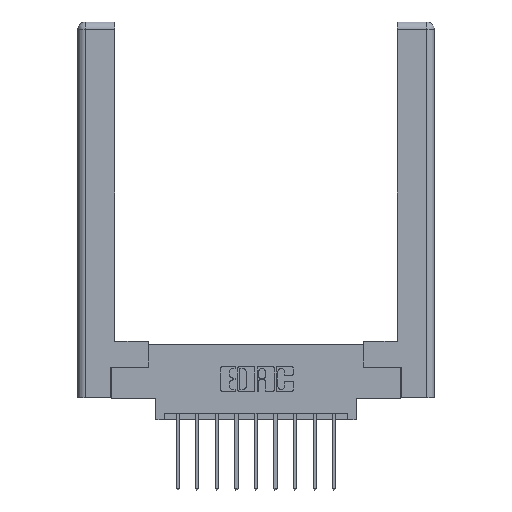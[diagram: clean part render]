
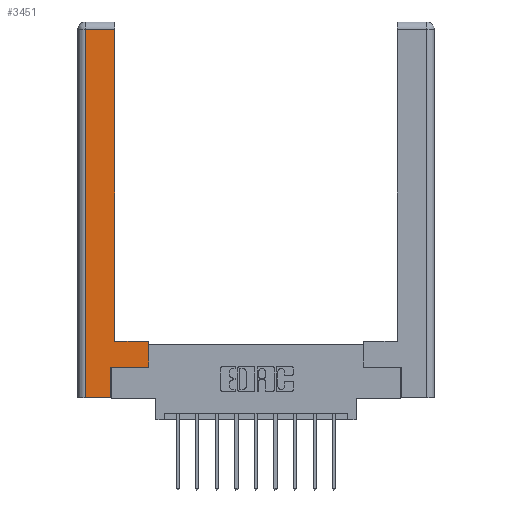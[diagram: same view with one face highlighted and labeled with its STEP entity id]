
A CAD part, top view. The second image highlights one B-rep face of the part: STEP entity #3451.
In plain terms, the highlighted planar face has unit normal (0, 0, 1).
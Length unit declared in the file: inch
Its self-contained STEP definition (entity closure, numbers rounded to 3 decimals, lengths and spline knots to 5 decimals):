
#70 = ORIENTED_EDGE ( 'NONE', *, *, #8937, .T. ) ;
#324 = FACE_OUTER_BOUND ( 'NONE', #2742, .T. ) ;
#689 = PLANE ( 'NONE',  #3331 ) ;
#798 = CARTESIAN_POINT ( 'NONE',  ( 0.295, 0.45, 0. ) ) ;
#870 = ORIENTED_EDGE ( 'NONE', *, *, #9145, .T. ) ;
#1037 = ORIENTED_EDGE ( 'NONE', *, *, #11974, .T. ) ;
#1301 = CARTESIAN_POINT ( 'NONE',  ( 0.565, 0.245, 0. ) ) ;
#1412 = VECTOR ( 'NONE', #5843, 39.37008 ) ;
#1646 = CARTESIAN_POINT ( 'NONE',  ( 0., 0., 0. ) ) ;
#2191 = DIRECTION ( 'NONE',  ( -1., 0., 0. ) ) ;
#2213 = DIRECTION ( 'NONE',  ( -1., 0., 0. ) ) ;
#2419 = LINE ( 'NONE', #10620, #13935 ) ;
#2433 = LINE ( 'NONE', #7003, #1412 ) ;
#2742 = EDGE_LOOP ( 'NONE', ( #870, #13878, #9900, #4125, #12414, #70, #5429, #1037 ) ) ;
#2788 = DIRECTION ( 'NONE',  ( 0., 0., -1. ) ) ;
#3029 = EDGE_CURVE ( 'NONE', #13375, #9802, #7976, .T. ) ;
#3331 = AXIS2_PLACEMENT_3D ( 'NONE', #1646, #2788, #6015 ) ;
#3368 = VERTEX_POINT ( 'NONE', #7949 ) ;
#3451 = ADVANCED_FACE ( 'NONE', ( #324 ), #689, .F. ) ;
#3477 = CARTESIAN_POINT ( 'NONE',  ( 0.265, 0.245, 0. ) ) ;
#3495 = CARTESIAN_POINT ( 'NONE',  ( 0.0615, 2.94, 0. ) ) ;
#4073 = VECTOR ( 'NONE', #6215, 39.37008 ) ;
#4125 = ORIENTED_EDGE ( 'NONE', *, *, #5815, .T. ) ;
#4282 = LINE ( 'NONE', #7533, #5321 ) ;
#4305 = EDGE_CURVE ( 'NONE', #12855, #12169, #7077, .T. ) ;
#4863 = LINE ( 'NONE', #11932, #9447 ) ;
#5131 = CARTESIAN_POINT ( 'NONE',  ( 0.565, 0.45, 0. ) ) ;
#5321 = VECTOR ( 'NONE', #2191, 39.37008 ) ;
#5429 = ORIENTED_EDGE ( 'NONE', *, *, #3029, .T. ) ;
#5466 = CARTESIAN_POINT ( 'NONE',  ( 0.265, 0.245, 0. ) ) ;
#5470 = LINE ( 'NONE', #3477, #13266 ) ;
#5790 = CARTESIAN_POINT ( 'NONE',  ( 0.295, 2.94, 0. ) ) ;
#5815 = EDGE_CURVE ( 'NONE', #9637, #3368, #9301, .T. ) ;
#5843 = DIRECTION ( 'NONE',  ( 1., 0., 0. ) ) ;
#6015 = DIRECTION ( 'NONE',  ( -1., 0., 0. ) ) ;
#6215 = DIRECTION ( 'NONE',  ( 0., 1., 0. ) ) ;
#6300 = DIRECTION ( 'NONE',  ( 0., 1., 0. ) ) ;
#6373 = CARTESIAN_POINT ( 'NONE',  ( 0.565, 0.45, 0. ) ) ;
#6769 = EDGE_CURVE ( 'NONE', #12169, #9637, #4863, .T. ) ;
#7003 = CARTESIAN_POINT ( 'NONE',  ( 0.565, 0.245, 0. ) ) ;
#7077 = LINE ( 'NONE', #8714, #12514 ) ;
#7533 = CARTESIAN_POINT ( 'NONE',  ( 0.295, 0.45, 0. ) ) ;
#7949 = CARTESIAN_POINT ( 'NONE',  ( 0.265, 0., 0. ) ) ;
#7976 = LINE ( 'NONE', #5131, #4073 ) ;
#8403 = VERTEX_POINT ( 'NONE', #798 ) ;
#8644 = VERTEX_POINT ( 'NONE', #5466 ) ;
#8714 = CARTESIAN_POINT ( 'NONE',  ( 0.0615, 2.94, 0. ) ) ;
#8937 = EDGE_CURVE ( 'NONE', #8644, #13375, #2433, .T. ) ;
#8974 = VECTOR ( 'NONE', #11617, 39.37008 ) ;
#9145 = EDGE_CURVE ( 'NONE', #8403, #12855, #2419, .T. ) ;
#9301 = LINE ( 'NONE', #10430, #8974 ) ;
#9407 = CARTESIAN_POINT ( 'NONE',  ( 0.0615, 0., 0. ) ) ;
#9447 = VECTOR ( 'NONE', #11770, 39.37008 ) ;
#9637 = VERTEX_POINT ( 'NONE', #9407 ) ;
#9802 = VERTEX_POINT ( 'NONE', #6373 ) ;
#9900 = ORIENTED_EDGE ( 'NONE', *, *, #6769, .T. ) ;
#10014 = DIRECTION ( 'NONE',  ( 0., 1., 0. ) ) ;
#10430 = CARTESIAN_POINT ( 'NONE',  ( 0.265, 0., 0. ) ) ;
#10620 = CARTESIAN_POINT ( 'NONE',  ( 0.295, 3., 0. ) ) ;
#11617 = DIRECTION ( 'NONE',  ( 1., 0., 0. ) ) ;
#11770 = DIRECTION ( 'NONE',  ( 0., -1., 0. ) ) ;
#11932 = CARTESIAN_POINT ( 'NONE',  ( 0.0615, 0., 0. ) ) ;
#11974 = EDGE_CURVE ( 'NONE', #9802, #8403, #4282, .T. ) ;
#12169 = VERTEX_POINT ( 'NONE', #3495 ) ;
#12414 = ORIENTED_EDGE ( 'NONE', *, *, #12772, .T. ) ;
#12514 = VECTOR ( 'NONE', #2213, 39.37008 ) ;
#12772 = EDGE_CURVE ( 'NONE', #3368, #8644, #5470, .T. ) ;
#12855 = VERTEX_POINT ( 'NONE', #5790 ) ;
#13266 = VECTOR ( 'NONE', #10014, 39.37008 ) ;
#13375 = VERTEX_POINT ( 'NONE', #1301 ) ;
#13878 = ORIENTED_EDGE ( 'NONE', *, *, #4305, .T. ) ;
#13935 = VECTOR ( 'NONE', #6300, 39.37008 ) ;
